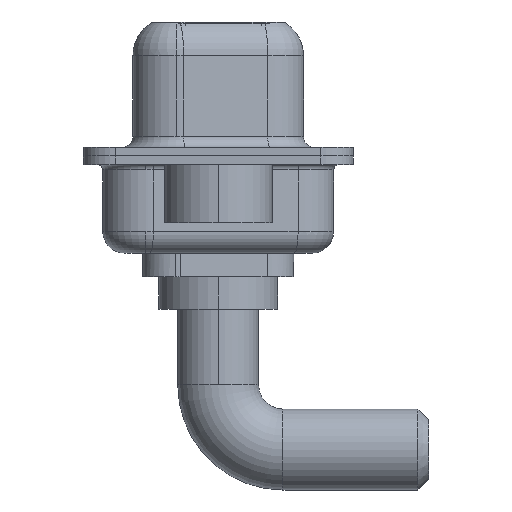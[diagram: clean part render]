
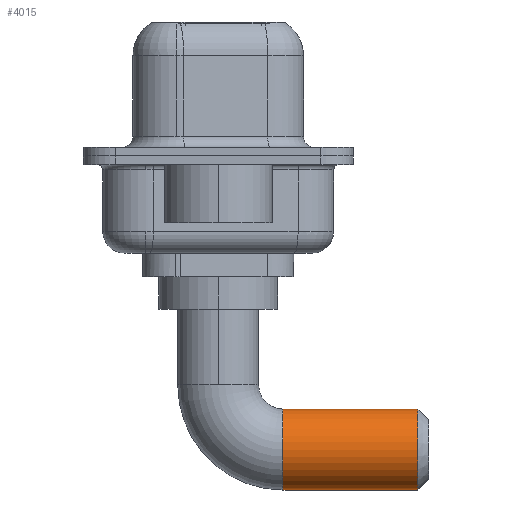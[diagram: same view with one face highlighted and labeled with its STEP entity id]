
A CAD part, left-side view. The second image highlights one B-rep face of the part: STEP entity #4015.
In plain terms, the highlighted cylindrical face has radius 1.875 mm (diameter 3.75 mm), a partial arc.
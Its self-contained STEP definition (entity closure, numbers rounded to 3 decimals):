
#310 = CARTESIAN_POINT ( 'NONE',  ( 0., -3., -6.5 ) ) ;
#372 = DIRECTION ( 'NONE',  ( -1., 0., 0. ) ) ;
#557 = VECTOR ( 'NONE', #7281, 1000. ) ;
#698 = VERTEX_POINT ( 'NONE', #4750 ) ;
#1138 = ORIENTED_EDGE ( 'NONE', *, *, #7909, .T. ) ;
#1527 = DIRECTION ( 'NONE',  ( 0., -1., 0. ) ) ;
#1774 = VECTOR ( 'NONE', #4762, 1000. ) ;
#2322 = AXIS2_PLACEMENT_3D ( 'NONE', #10369, #10431, #3772 ) ;
#2460 = CARTESIAN_POINT ( 'NONE',  ( 0., -3., -6.5 ) ) ;
#2816 = CARTESIAN_POINT ( 'NONE',  ( 0., -3., -4.625 ) ) ;
#3469 = CARTESIAN_POINT ( 'NONE',  ( 0., -3., -8.375 ) ) ;
#3630 = VERTEX_POINT ( 'NONE', #10424 ) ;
#3667 = VERTEX_POINT ( 'NONE', #10849 ) ;
#3772 = DIRECTION ( 'NONE',  ( 0., 0., -1. ) ) ;
#4015 = ADVANCED_FACE ( 'NONE', ( #4282 ), #12008, .T. ) ;
#4222 = LINE ( 'NONE', #12124, #557 ) ;
#4282 = FACE_OUTER_BOUND ( 'NONE', #6179, .T. ) ;
#4750 = CARTESIAN_POINT ( 'NONE',  ( 0., -3., -4.625 ) ) ;
#4762 = DIRECTION ( 'NONE',  ( 0., -1., 0. ) ) ;
#6179 = EDGE_LOOP ( 'NONE', ( #8636, #8062, #11711, #1138 ) ) ;
#6472 = DIRECTION ( 'NONE',  ( 0., 0., -1. ) ) ;
#7243 = AXIS2_PLACEMENT_3D ( 'NONE', #2460, #1527, #6472 ) ;
#7281 = DIRECTION ( 'NONE',  ( 0., -1., 0. ) ) ;
#7909 = EDGE_CURVE ( 'NONE', #3667, #3630, #10936, .T. ) ;
#7963 = DIRECTION ( 'NONE',  ( 0., -1., 0. ) ) ;
#8062 = ORIENTED_EDGE ( 'NONE', *, *, #9225, .T. ) ;
#8327 = CIRCLE ( 'NONE', #12125, 1.875 ) ;
#8636 = ORIENTED_EDGE ( 'NONE', *, *, #12389, .F. ) ;
#9225 = EDGE_CURVE ( 'NONE', #698, #11781, #8327, .T. ) ;
#10369 = CARTESIAN_POINT ( 'NONE',  ( 0., -9.25, -6.5 ) ) ;
#10424 = CARTESIAN_POINT ( 'NONE',  ( 0., -9.25, -4.625 ) ) ;
#10431 = DIRECTION ( 'NONE',  ( 0., 1., 0. ) ) ;
#10849 = CARTESIAN_POINT ( 'NONE',  ( 0., -9.25, -8.375 ) ) ;
#10936 = CIRCLE ( 'NONE', #2322, 1.875 ) ;
#11426 = LINE ( 'NONE', #2816, #1774 ) ;
#11706 = EDGE_CURVE ( 'NONE', #11781, #3667, #4222, .T. ) ;
#11711 = ORIENTED_EDGE ( 'NONE', *, *, #11706, .T. ) ;
#11781 = VERTEX_POINT ( 'NONE', #3469 ) ;
#12008 = CYLINDRICAL_SURFACE ( 'NONE', #7243, 1.875 ) ;
#12124 = CARTESIAN_POINT ( 'NONE',  ( 0., -3., -8.375 ) ) ;
#12125 = AXIS2_PLACEMENT_3D ( 'NONE', #310, #7963, #372 ) ;
#12389 = EDGE_CURVE ( 'NONE', #698, #3630, #11426, .T. ) ;
